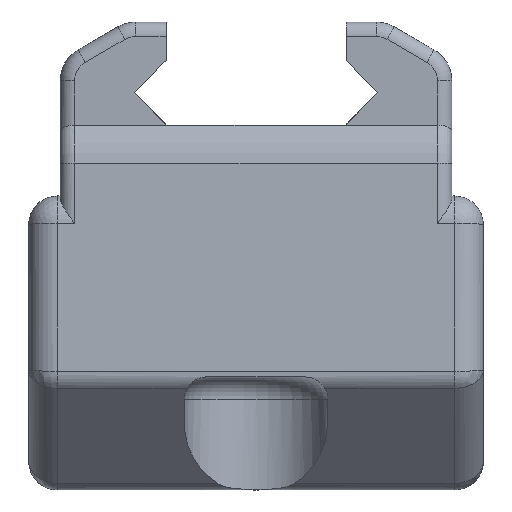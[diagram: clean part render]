
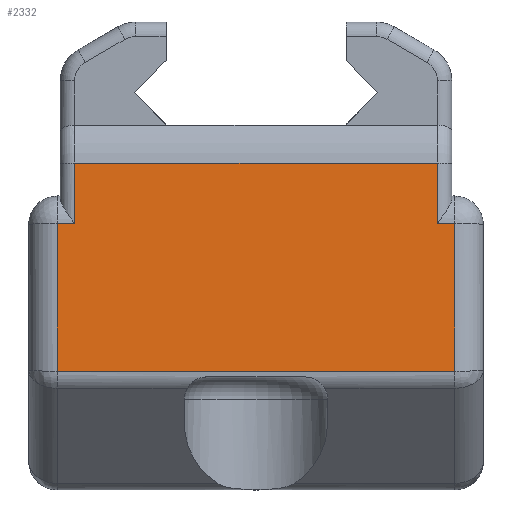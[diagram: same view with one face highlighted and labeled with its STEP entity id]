
A CAD part, front view. The second image highlights one B-rep face of the part: STEP entity #2332.
In plain terms, the highlighted planar face has unit normal (0, -0.999, 0.044).
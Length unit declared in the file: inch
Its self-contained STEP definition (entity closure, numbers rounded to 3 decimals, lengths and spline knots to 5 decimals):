
#53=PLANE('',#2519);
#175=FACE_OUTER_BOUND('',#314,.T.);
#314=EDGE_LOOP('',(#1727,#1728,#1729,#1730,#1731,#1732,#1733,#1734));
#618=LINE('',#10021,#817);
#619=LINE('',#10024,#818);
#623=LINE('',#10034,#822);
#624=LINE('',#10036,#823);
#625=LINE('',#10038,#824);
#626=LINE('',#10040,#825);
#627=LINE('',#10042,#826);
#628=LINE('',#10043,#827);
#817=VECTOR('',#2889,0.3937);
#818=VECTOR('',#2892,0.3937);
#822=VECTOR('',#2900,0.3937);
#823=VECTOR('',#2901,0.3937);
#824=VECTOR('',#2902,0.3937);
#825=VECTOR('',#2903,0.3937);
#826=VECTOR('',#2904,0.3937);
#827=VECTOR('',#2905,0.3937);
#1060=VERTEX_POINT('',#9976);
#1062=VERTEX_POINT('',#10010);
#1063=VERTEX_POINT('',#10023);
#1067=VERTEX_POINT('',#10033);
#1068=VERTEX_POINT('',#10035);
#1069=VERTEX_POINT('',#10037);
#1070=VERTEX_POINT('',#10039);
#1071=VERTEX_POINT('',#10041);
#1308=EDGE_CURVE('',#1062,#1060,#618,.T.);
#1309=EDGE_CURVE('',#1063,#1060,#619,.T.);
#1314=EDGE_CURVE('',#1067,#1062,#623,.T.);
#1315=EDGE_CURVE('',#1068,#1067,#624,.T.);
#1316=EDGE_CURVE('',#1069,#1068,#625,.T.);
#1317=EDGE_CURVE('',#1070,#1069,#626,.T.);
#1318=EDGE_CURVE('',#1071,#1070,#627,.T.);
#1319=EDGE_CURVE('',#1063,#1071,#628,.T.);
#1727=ORIENTED_EDGE('',*,*,#1308,.F.);
#1728=ORIENTED_EDGE('',*,*,#1314,.F.);
#1729=ORIENTED_EDGE('',*,*,#1315,.F.);
#1730=ORIENTED_EDGE('',*,*,#1316,.F.);
#1731=ORIENTED_EDGE('',*,*,#1317,.F.);
#1732=ORIENTED_EDGE('',*,*,#1318,.F.);
#1733=ORIENTED_EDGE('',*,*,#1319,.F.);
#1734=ORIENTED_EDGE('',*,*,#1309,.T.);
#2332=ADVANCED_FACE('',(#175),#53,.T.);
#2519=AXIS2_PLACEMENT_3D('',#10032,#2898,#2899);
#2889=DIRECTION('',(0.,0.044,0.999));
#2892=DIRECTION('',(-1.,0.,0.));
#2898=DIRECTION('center_axis',(0.,-0.999,
0.044));
#2899=DIRECTION('ref_axis',(0.,0.044,0.999));
#2900=DIRECTION('',(1.,0.,0.));
#2901=DIRECTION('',(0.,0.044,0.999));
#2902=DIRECTION('',(-1.,0.,0.));
#2903=DIRECTION('',(0.,-0.044,-0.999));
#2904=DIRECTION('',(1.,0.,0.));
#2905=DIRECTION('',(0.,-0.044,-0.999));
#9976=CARTESIAN_POINT('',(-0.64655,-0.74752,0.75979));
#10010=CARTESIAN_POINT('',(-0.64655,-0.75689,0.54948));
#10021=CARTESIAN_POINT('',(-0.64655,-0.56772,4.79702));
#10023=CARTESIAN_POINT('',(0.6172,-0.74752,0.75979));
#10024=CARTESIAN_POINT('',(0.32618,-0.74752,0.75979));
#10032=CARTESIAN_POINT('Origin',(-0.01484,-0.39823,
8.60287));
#10033=CARTESIAN_POINT('',(-0.70617,-0.75689,0.54948));
#10034=CARTESIAN_POINT('',(-0.11917,-0.75689,0.54948));
#10035=CARTESIAN_POINT('',(-0.70617,-0.7798,0.03487));
#10036=CARTESIAN_POINT('',(-0.70617,-0.60876,3.87558));
#10037=CARTESIAN_POINT('',(0.6765,-0.7798,0.03487));
#10038=CARTESIAN_POINT('',(-0.24318,-0.7798,0.03487));
#10039=CARTESIAN_POINT('',(0.6765,-0.75689,0.54948));
#10040=CARTESIAN_POINT('',(0.6765,-0.57354,4.66634));
#10041=CARTESIAN_POINT('',(0.6172,-0.75689,0.54948));
#10042=CARTESIAN_POINT('',(-0.11917,-0.75689,0.54948));
#10043=CARTESIAN_POINT('',(0.6172,-0.56772,4.79702));
